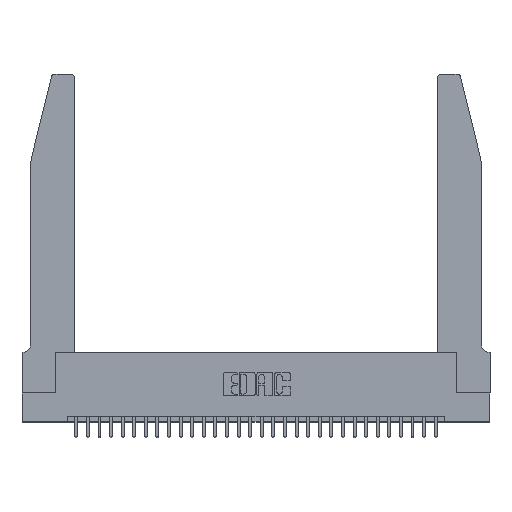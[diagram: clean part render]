
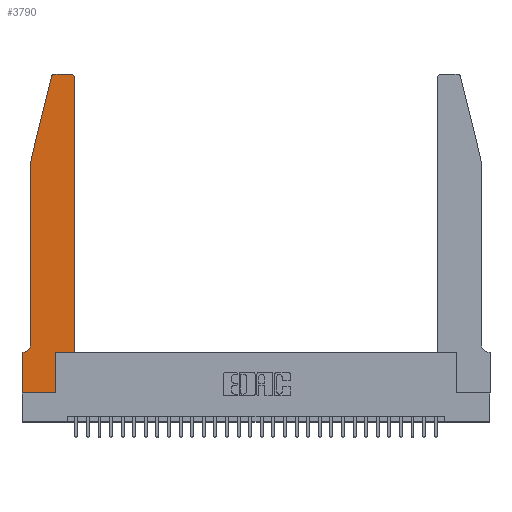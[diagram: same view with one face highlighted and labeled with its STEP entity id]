
A CAD part, top view. The second image highlights one B-rep face of the part: STEP entity #3790.
In plain terms, the highlighted planar face has unit normal (0, 0, 1).
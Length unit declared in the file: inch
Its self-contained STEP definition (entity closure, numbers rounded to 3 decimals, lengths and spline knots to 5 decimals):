
#373 = ORIENTED_EDGE ( 'NONE', *, *, #10974, .T. ) ;
#1140 = CARTESIAN_POINT ( 'NONE',  ( 0.4205, 2.72, 0.37 ) ) ;
#1499 = CARTESIAN_POINT ( 'NONE',  ( 0.4505, 0.35, 0.37 ) ) ;
#1648 = DIRECTION ( 'NONE',  ( 0., 0., 1. ) ) ;
#1996 = LINE ( 'NONE', #15040, #31062 ) ;
#2071 = VERTEX_POINT ( 'NONE', #5044 ) ;
#2379 = EDGE_LOOP ( 'NONE', ( #2742, #5917, #9723, #3344, #29064, #12340, #27275, #27338, #14031, #19353, #15053, #373 ) ) ;
#2742 = ORIENTED_EDGE ( 'NONE', *, *, #18275, .T. ) ;
#2798 = FACE_OUTER_BOUND ( 'NONE', #2379, .T. ) ;
#2808 = EDGE_CURVE ( 'NONE', #2071, #9028, #17114, .T. ) ;
#3344 = ORIENTED_EDGE ( 'NONE', *, *, #29493, .T. ) ;
#3775 = VECTOR ( 'NONE', #17782, 39.37008 ) ;
#3790 = ADVANCED_FACE ( 'NONE', ( #2798 ), #6355, .T. ) ;
#3968 = VERTEX_POINT ( 'NONE', #18113 ) ;
#4209 = CARTESIAN_POINT ( 'NONE',  ( 0.284, 2.72, 0.37 ) ) ;
#4359 = AXIS2_PLACEMENT_3D ( 'NONE', #4209, #23534, #15785 ) ;
#4741 = VERTEX_POINT ( 'NONE', #28684 ) ;
#5044 = CARTESIAN_POINT ( 'NONE',  ( 0.4505, 0.35, 0.37 ) ) ;
#5473 = AXIS2_PLACEMENT_3D ( 'NONE', #17282, #24313, #27146 ) ;
#5631 = LINE ( 'NONE', #30295, #3775 ) ;
#5662 = CARTESIAN_POINT ( 'NONE',  ( 0., 0., 0.37 ) ) ;
#5917 = ORIENTED_EDGE ( 'NONE', *, *, #7766, .T. ) ;
#6029 = CARTESIAN_POINT ( 'NONE',  ( 0.0755, 0.35, 0.37 ) ) ;
#6355 = PLANE ( 'NONE',  #20693 ) ;
#6358 = LINE ( 'NONE', #9446, #14256 ) ;
#6719 = VERTEX_POINT ( 'NONE', #15572 ) ;
#7766 = EDGE_CURVE ( 'NONE', #6719, #4741, #12719, .T. ) ;
#7773 = VERTEX_POINT ( 'NONE', #5662 ) ;
#8430 = DIRECTION ( 'NONE',  ( -1., 0., 0. ) ) ;
#9028 = VERTEX_POINT ( 'NONE', #13282 ) ;
#9446 = CARTESIAN_POINT ( 'NONE',  ( 0.2865, 0.35, 0.37 ) ) ;
#9599 = DIRECTION ( 'NONE',  ( -1., 0., 0. ) ) ;
#9661 = DIRECTION ( 'NONE',  ( 0., 1., 0. ) ) ;
#9723 = ORIENTED_EDGE ( 'NONE', *, *, #26896, .T. ) ;
#9853 = EDGE_CURVE ( 'NONE', #14696, #13802, #13604, .T. ) ;
#9959 = VECTOR ( 'NONE', #19701, 39.37008 ) ;
#10043 = CARTESIAN_POINT ( 'NONE',  ( 0.0055, 0.35, 0.37 ) ) ;
#10488 = LINE ( 'NONE', #17715, #24139 ) ;
#10974 = EDGE_CURVE ( 'NONE', #9028, #23170, #15420, .T. ) ;
#11088 = VERTEX_POINT ( 'NONE', #15857 ) ;
#11301 = LINE ( 'NONE', #1499, #24915 ) ;
#11468 = EDGE_CURVE ( 'NONE', #7773, #3968, #10488, .T. ) ;
#11924 = CARTESIAN_POINT ( 'NONE',  ( 0.2865, 0.35, 0.37 ) ) ;
#12124 = CARTESIAN_POINT ( 'NONE',  ( 0.2605, 2.75, 0.37 ) ) ;
#12340 = ORIENTED_EDGE ( 'NONE', *, *, #9853, .T. ) ;
#12719 = CIRCLE ( 'NONE', #4359, 0.03 ) ;
#12862 = DIRECTION ( 'NONE',  ( 1., 0., 0. ) ) ;
#12951 = VECTOR ( 'NONE', #9599, 39.37008 ) ;
#13282 = CARTESIAN_POINT ( 'NONE',  ( 0.4505, 2.72, 0.37 ) ) ;
#13604 = LINE ( 'NONE', #6029, #29131 ) ;
#13802 = VERTEX_POINT ( 'NONE', #28714 ) ;
#14031 = ORIENTED_EDGE ( 'NONE', *, *, #15892, .T. ) ;
#14256 = VECTOR ( 'NONE', #9661, 39.37008 ) ;
#14496 = AXIS2_PLACEMENT_3D ( 'NONE', #1140, #27403, #30167 ) ;
#14696 = VERTEX_POINT ( 'NONE', #10043 ) ;
#15040 = CARTESIAN_POINT ( 'NONE',  ( 0.0755, 2., 0.37 ) ) ;
#15053 = ORIENTED_EDGE ( 'NONE', *, *, #2808, .T. ) ;
#15275 = DIRECTION ( 'NONE',  ( 1., 0., 0. ) ) ;
#15420 = CIRCLE ( 'NONE', #14496, 0.03 ) ;
#15572 = CARTESIAN_POINT ( 'NONE',  ( 0.284, 2.75, 0.37 ) ) ;
#15785 = DIRECTION ( 'NONE',  ( 1., 0., 0. ) ) ;
#15857 = CARTESIAN_POINT ( 'NONE',  ( 0.0755, 2., 0.37 ) ) ;
#15892 = EDGE_CURVE ( 'NONE', #3968, #30902, #6358, .T. ) ;
#16973 = VECTOR ( 'NONE', #19062, 39.37008 ) ;
#17114 = LINE ( 'NONE', #29552, #9959 ) ;
#17282 = CARTESIAN_POINT ( 'NONE',  ( 0.0055, 0.42, 0.37 ) ) ;
#17715 = CARTESIAN_POINT ( 'NONE',  ( 0., 0., 0.37 ) ) ;
#17782 = DIRECTION ( 'NONE',  ( 0., -1., 0. ) ) ;
#18113 = CARTESIAN_POINT ( 'NONE',  ( 0.2865, 0., 0.37 ) ) ;
#18275 = EDGE_CURVE ( 'NONE', #23170, #6719, #22446, .T. ) ;
#18726 = CARTESIAN_POINT ( 'NONE',  ( 0.0755, 0.42, 0.37 ) ) ;
#19062 = DIRECTION ( 'NONE',  ( 0., -1., 0. ) ) ;
#19353 = ORIENTED_EDGE ( 'NONE', *, *, #29590, .T. ) ;
#19407 = VERTEX_POINT ( 'NONE', #18726 ) ;
#19701 = DIRECTION ( 'NONE',  ( 0., 1., 0. ) ) ;
#20693 = AXIS2_PLACEMENT_3D ( 'NONE', #20721, #1648, #15275 ) ;
#20721 = CARTESIAN_POINT ( 'NONE',  ( 0., 0.35, 0.37 ) ) ;
#21081 = CARTESIAN_POINT ( 'NONE',  ( 0.4205, 2.75, 0.37 ) ) ;
#21632 = CARTESIAN_POINT ( 'NONE',  ( 0., 0., 0.37 ) ) ;
#22446 = LINE ( 'NONE', #12124, #12951 ) ;
#23113 = DIRECTION ( 'NONE',  ( -0.239, -0.971, 0. ) ) ;
#23170 = VERTEX_POINT ( 'NONE', #21081 ) ;
#23534 = DIRECTION ( 'NONE',  ( 0., 0., 1. ) ) ;
#24139 = VECTOR ( 'NONE', #12862, 39.37008 ) ;
#24313 = DIRECTION ( 'NONE',  ( 0., 0., -1. ) ) ;
#24353 = CIRCLE ( 'NONE', #5473, 0.07 ) ;
#24915 = VECTOR ( 'NONE', #25739, 39.37008 ) ;
#25272 = EDGE_CURVE ( 'NONE', #19407, #14696, #24353, .T. ) ;
#25739 = DIRECTION ( 'NONE',  ( 1., 0., 0. ) ) ;
#26896 = EDGE_CURVE ( 'NONE', #4741, #11088, #1996, .T. ) ;
#27146 = DIRECTION ( 'NONE',  ( -1., 0., 0. ) ) ;
#27275 = ORIENTED_EDGE ( 'NONE', *, *, #27869, .T. ) ;
#27338 = ORIENTED_EDGE ( 'NONE', *, *, #11468, .T. ) ;
#27403 = DIRECTION ( 'NONE',  ( 0., 0., 1. ) ) ;
#27869 = EDGE_CURVE ( 'NONE', #13802, #7773, #29126, .T. ) ;
#28684 = CARTESIAN_POINT ( 'NONE',  ( 0.25487, 2.72718, 0.37 ) ) ;
#28714 = CARTESIAN_POINT ( 'NONE',  ( 0., 0.35, 0.37 ) ) ;
#29064 = ORIENTED_EDGE ( 'NONE', *, *, #25272, .T. ) ;
#29126 = LINE ( 'NONE', #21632, #16973 ) ;
#29131 = VECTOR ( 'NONE', #8430, 39.37008 ) ;
#29493 = EDGE_CURVE ( 'NONE', #11088, #19407, #5631, .T. ) ;
#29552 = CARTESIAN_POINT ( 'NONE',  ( 0.4505, 0.35, 0.37 ) ) ;
#29590 = EDGE_CURVE ( 'NONE', #30902, #2071, #11301, .T. ) ;
#30167 = DIRECTION ( 'NONE',  ( 1., 0., 0. ) ) ;
#30295 = CARTESIAN_POINT ( 'NONE',  ( 0.0755, 2., 0.37 ) ) ;
#30902 = VERTEX_POINT ( 'NONE', #11924 ) ;
#31062 = VECTOR ( 'NONE', #23113, 39.37008 ) ;
